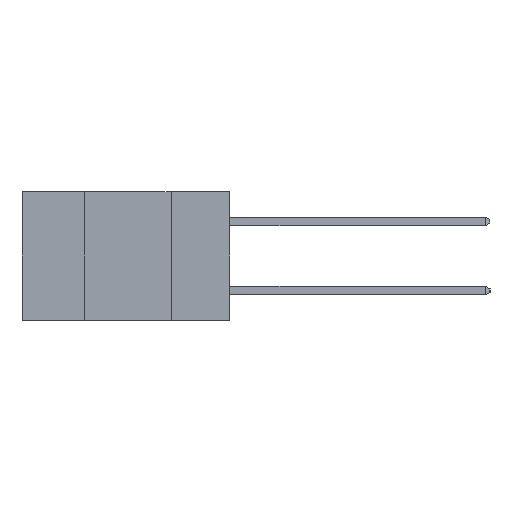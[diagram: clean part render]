
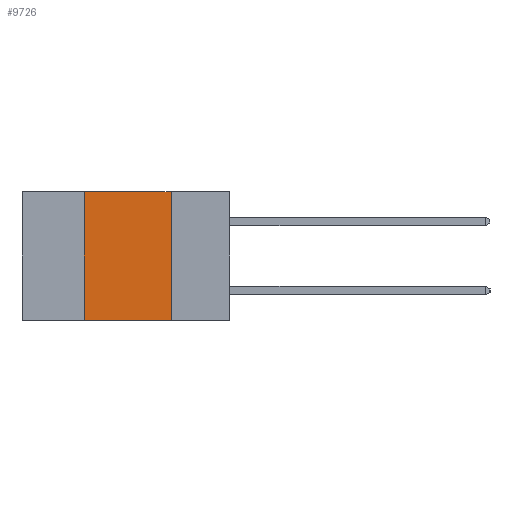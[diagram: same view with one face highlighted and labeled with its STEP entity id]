
A CAD part, left-side view. The second image highlights one B-rep face of the part: STEP entity #9726.
In plain terms, the highlighted planar face has unit normal (-1, 0, 0).
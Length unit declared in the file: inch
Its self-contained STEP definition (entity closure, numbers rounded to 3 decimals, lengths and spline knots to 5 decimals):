
#773 = VERTEX_POINT ( 'NONE', #3414 ) ;
#973 = LINE ( 'NONE', #8346, #10454 ) ;
#1137 = ORIENTED_EDGE ( 'NONE', *, *, #4623, .T. ) ;
#1957 = AXIS2_PLACEMENT_3D ( 'NONE', #8623, #8598, #8588 ) ;
#2027 = VECTOR ( 'NONE', #8498, 39.37008 ) ;
#2696 = VERTEX_POINT ( 'NONE', #5181 ) ;
#2747 = VECTOR ( 'NONE', #11583, 39.37008 ) ;
#3414 = CARTESIAN_POINT ( 'NONE',  ( 0., 0.17, -0.37 ) ) ;
#3756 = ORIENTED_EDGE ( 'NONE', *, *, #5819, .F. ) ;
#4115 = VERTEX_POINT ( 'NONE', #11644 ) ;
#4385 = EDGE_CURVE ( 'NONE', #11992, #773, #10315, .T. ) ;
#4623 = EDGE_CURVE ( 'NONE', #4115, #773, #973, .T. ) ;
#4707 = LINE ( 'NONE', #11560, #2747 ) ;
#5181 = CARTESIAN_POINT ( 'NONE',  ( 0., 0.42, 0. ) ) ;
#5819 = EDGE_CURVE ( 'NONE', #2696, #11992, #9560, .T. ) ;
#5926 = ORIENTED_EDGE ( 'NONE', *, *, #4385, .F. ) ;
#7746 = CARTESIAN_POINT ( 'NONE',  ( 0., 0.6, 0. ) ) ;
#7774 = EDGE_LOOP ( 'NONE', ( #5926, #3756, #8270, #1137 ) ) ;
#7836 = VECTOR ( 'NONE', #9707, 39.37008 ) ;
#8152 = DIRECTION ( 'NONE',  ( 0., -1., 0. ) ) ;
#8270 = ORIENTED_EDGE ( 'NONE', *, *, #8582, .F. ) ;
#8346 = CARTESIAN_POINT ( 'NONE',  ( 0., 0.6, -0.37 ) ) ;
#8498 = DIRECTION ( 'NONE',  ( 0., -1., 0. ) ) ;
#8582 = EDGE_CURVE ( 'NONE', #4115, #2696, #4707, .T. ) ;
#8588 = DIRECTION ( 'NONE',  ( 0., 0., -1. ) ) ;
#8593 = FACE_OUTER_BOUND ( 'NONE', #7774, .T. ) ;
#8598 = DIRECTION ( 'NONE',  ( 1., 0., 0. ) ) ;
#8623 = CARTESIAN_POINT ( 'NONE',  ( 0., 0.6, 0. ) ) ;
#8706 = PLANE ( 'NONE',  #1957 ) ;
#9133 = CARTESIAN_POINT ( 'NONE',  ( 0., 0.17, 0. ) ) ;
#9560 = LINE ( 'NONE', #7746, #2027 ) ;
#9707 = DIRECTION ( 'NONE',  ( 0., 0., -1. ) ) ;
#9726 = ADVANCED_FACE ( 'NONE', ( #8593 ), #8706, .F. ) ;
#9749 = CARTESIAN_POINT ( 'NONE',  ( 0., 0.17, -0.37 ) ) ;
#10315 = LINE ( 'NONE', #9749, #7836 ) ;
#10454 = VECTOR ( 'NONE', #8152, 39.37008 ) ;
#11560 = CARTESIAN_POINT ( 'NONE',  ( 0., 0.42, -0.37 ) ) ;
#11583 = DIRECTION ( 'NONE',  ( 0., 0., 1. ) ) ;
#11644 = CARTESIAN_POINT ( 'NONE',  ( 0., 0.42, -0.37 ) ) ;
#11992 = VERTEX_POINT ( 'NONE', #9133 ) ;
